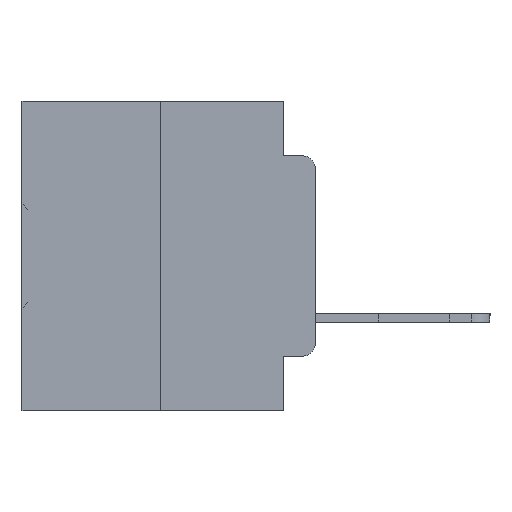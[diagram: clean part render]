
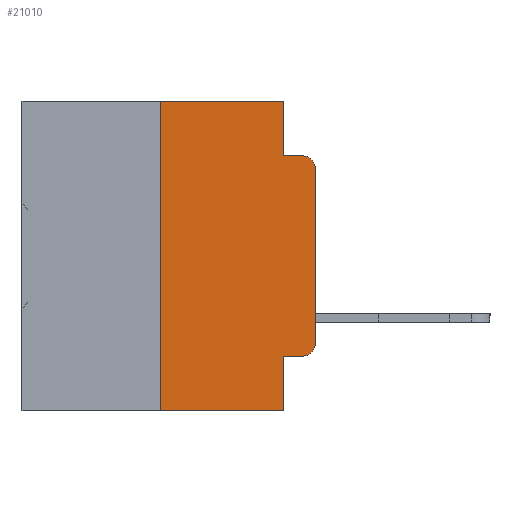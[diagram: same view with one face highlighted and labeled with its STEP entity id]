
A CAD part, left-side view. The second image highlights one B-rep face of the part: STEP entity #21010.
In plain terms, the highlighted planar face has unit normal (-1, 0, 0).
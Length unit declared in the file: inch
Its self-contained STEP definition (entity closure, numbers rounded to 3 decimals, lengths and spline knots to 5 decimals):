
#525 = ORIENTED_EDGE ( 'NONE', *, *, #20461, .F. ) ;
#891 = ORIENTED_EDGE ( 'NONE', *, *, #32799, .T. ) ;
#1102 = VERTEX_POINT ( 'NONE', #30756 ) ;
#1128 = VECTOR ( 'NONE', #18170, 39.37008 ) ;
#1728 = CARTESIAN_POINT ( 'NONE',  ( 0., 0.051, 0. ) ) ;
#2946 = LINE ( 'NONE', #1728, #10396 ) ;
#4136 = CARTESIAN_POINT ( 'NONE',  ( 0., 0.02, -0.0885 ) ) ;
#4517 = DIRECTION ( 'NONE',  ( 0., 0., -1. ) ) ;
#4996 = LINE ( 'NONE', #27773, #19025 ) ;
#5680 = AXIS2_PLACEMENT_3D ( 'NONE', #11829, #31331, #14654 ) ;
#6157 = VERTEX_POINT ( 'NONE', #4136 ) ;
#6400 = EDGE_CURVE ( 'NONE', #14929, #26730, #25868, .T. ) ;
#6995 = LINE ( 'NONE', #23769, #35798 ) ;
#7018 = DIRECTION ( 'NONE',  ( 0., -1., 0. ) ) ;
#8787 = ORIENTED_EDGE ( 'NONE', *, *, #30937, .T. ) ;
#9189 = EDGE_CURVE ( 'NONE', #12738, #1102, #15948, .T. ) ;
#9597 = DIRECTION ( 'NONE',  ( 0., -1., 0. ) ) ;
#10121 = VECTOR ( 'NONE', #24908, 39.37008 ) ;
#10396 = VECTOR ( 'NONE', #4517, 39.37008 ) ;
#10902 = VECTOR ( 'NONE', #18557, 39.37008 ) ;
#11259 = PLANE ( 'NONE',  #36115 ) ;
#11264 = CARTESIAN_POINT ( 'NONE',  ( 0., 0.051, -0.0885 ) ) ;
#11829 = CARTESIAN_POINT ( 'NONE',  ( 0., 0.02, -0.3915 ) ) ;
#12020 = ORIENTED_EDGE ( 'NONE', *, *, #18589, .F. ) ;
#12492 = ORIENTED_EDGE ( 'NONE', *, *, #16691, .T. ) ;
#12738 = VERTEX_POINT ( 'NONE', #29622 ) ;
#13238 = DIRECTION ( 'NONE',  ( 0., 0., -1. ) ) ;
#14099 = DIRECTION ( 'NONE',  ( 1., 0., 0. ) ) ;
#14607 = FACE_OUTER_BOUND ( 'NONE', #24833, .T. ) ;
#14654 = DIRECTION ( 'NONE',  ( 0., 0., -1. ) ) ;
#14795 = VERTEX_POINT ( 'NONE', #25837 ) ;
#14929 = VERTEX_POINT ( 'NONE', #21446 ) ;
#15372 = CARTESIAN_POINT ( 'NONE',  ( 0., 0.473, 0. ) ) ;
#15481 = ORIENTED_EDGE ( 'NONE', *, *, #6400, .T. ) ;
#15948 = CIRCLE ( 'NONE', #5680, 0.02 ) ;
#16064 = VECTOR ( 'NONE', #13238, 39.37008 ) ;
#16171 = DIRECTION ( 'NONE',  ( -1., 0., 0. ) ) ;
#16673 = DIRECTION ( 'NONE',  ( 0., 0., 1. ) ) ;
#16691 = EDGE_CURVE ( 'NONE', #21812, #12738, #6995, .T. ) ;
#16751 = AXIS2_PLACEMENT_3D ( 'NONE', #32856, #16171, #35669 ) ;
#17034 = VERTEX_POINT ( 'NONE', #11264 ) ;
#17322 = VERTEX_POINT ( 'NONE', #17995 ) ;
#17573 = CARTESIAN_POINT ( 'NONE',  ( 0., 0.051, -0.4115 ) ) ;
#17995 = CARTESIAN_POINT ( 'NONE',  ( 0., 0.25, 0. ) ) ;
#18170 = DIRECTION ( 'NONE',  ( 0., -1., 0. ) ) ;
#18557 = DIRECTION ( 'NONE',  ( 0., 0., 1. ) ) ;
#18589 = EDGE_CURVE ( 'NONE', #21812, #26730, #2946, .T. ) ;
#18601 = VERTEX_POINT ( 'NONE', #29687 ) ;
#19025 = VECTOR ( 'NONE', #16673, 39.37008 ) ;
#19322 = CARTESIAN_POINT ( 'NONE',  ( 0., 0.473, -0.5 ) ) ;
#19669 = LINE ( 'NONE', #23546, #27047 ) ;
#20233 = ORIENTED_EDGE ( 'NONE', *, *, #34730, .F. ) ;
#20461 = EDGE_CURVE ( 'NONE', #14929, #17322, #4996, .T. ) ;
#21010 = ADVANCED_FACE ( 'NONE', ( #14607 ), #11259, .F. ) ;
#21446 = CARTESIAN_POINT ( 'NONE',  ( 0., 0.25, -0.5 ) ) ;
#21812 = VERTEX_POINT ( 'NONE', #17573 ) ;
#22010 = CIRCLE ( 'NONE', #16751, 0.02 ) ;
#23496 = EDGE_CURVE ( 'NONE', #17034, #6157, #19669, .T. ) ;
#23509 = LINE ( 'NONE', #32601, #16064 ) ;
#23546 = CARTESIAN_POINT ( 'NONE',  ( 0., 0.051, -0.0885 ) ) ;
#23769 = CARTESIAN_POINT ( 'NONE',  ( 0., 0.051, -0.4115 ) ) ;
#24159 = CARTESIAN_POINT ( 'NONE',  ( 0., 0., 0. ) ) ;
#24414 = CARTESIAN_POINT ( 'NONE',  ( 0., 0.051, -0.5 ) ) ;
#24833 = EDGE_LOOP ( 'NONE', ( #891, #8787, #32788, #31504, #20233, #525, #15481, #12020, #12492, #29067 ) ) ;
#24908 = DIRECTION ( 'NONE',  ( 0., -1., 0. ) ) ;
#25837 = CARTESIAN_POINT ( 'NONE',  ( 0., 0.051, 0. ) ) ;
#25868 = LINE ( 'NONE', #19322, #10121 ) ;
#26730 = VERTEX_POINT ( 'NONE', #24414 ) ;
#27047 = VECTOR ( 'NONE', #9597, 39.37008 ) ;
#27773 = CARTESIAN_POINT ( 'NONE',  ( 0., 0.25, 0. ) ) ;
#27912 = EDGE_CURVE ( 'NONE', #14795, #17034, #23509, .T. ) ;
#27993 = CARTESIAN_POINT ( 'NONE',  ( 0., 0.473, 0. ) ) ;
#29067 = ORIENTED_EDGE ( 'NONE', *, *, #9189, .T. ) ;
#29622 = CARTESIAN_POINT ( 'NONE',  ( 0., 0.02, -0.4115 ) ) ;
#29687 = CARTESIAN_POINT ( 'NONE',  ( 0., 0., -0.1085 ) ) ;
#30756 = CARTESIAN_POINT ( 'NONE',  ( 0., 0., -0.3915 ) ) ;
#30832 = LINE ( 'NONE', #15372, #1128 ) ;
#30937 = EDGE_CURVE ( 'NONE', #18601, #6157, #22010, .T. ) ;
#31331 = DIRECTION ( 'NONE',  ( -1., 0., 0. ) ) ;
#31504 = ORIENTED_EDGE ( 'NONE', *, *, #27912, .F. ) ;
#32305 = LINE ( 'NONE', #24159, #10902 ) ;
#32601 = CARTESIAN_POINT ( 'NONE',  ( 0., 0.051, 0. ) ) ;
#32788 = ORIENTED_EDGE ( 'NONE', *, *, #23496, .F. ) ;
#32799 = EDGE_CURVE ( 'NONE', #1102, #18601, #32305, .T. ) ;
#32856 = CARTESIAN_POINT ( 'NONE',  ( 0., 0.02, -0.1085 ) ) ;
#33583 = DIRECTION ( 'NONE',  ( 0., 0., -1. ) ) ;
#34730 = EDGE_CURVE ( 'NONE', #17322, #14795, #30832, .T. ) ;
#35669 = DIRECTION ( 'NONE',  ( 0., 0., -1. ) ) ;
#35798 = VECTOR ( 'NONE', #7018, 39.37008 ) ;
#36115 = AXIS2_PLACEMENT_3D ( 'NONE', #27993, #14099, #33583 ) ;
